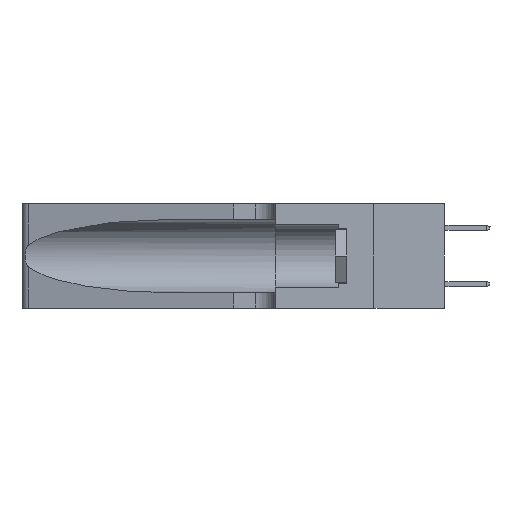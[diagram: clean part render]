
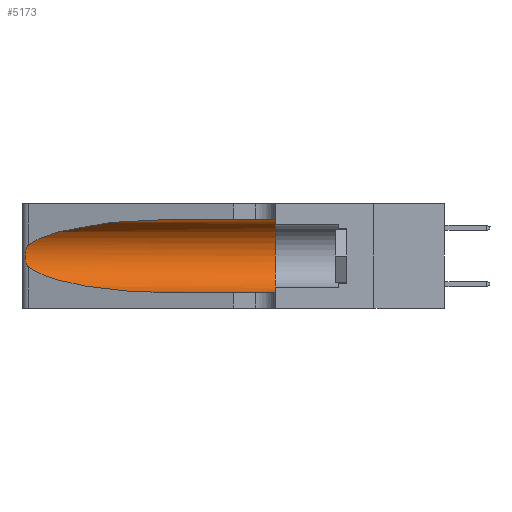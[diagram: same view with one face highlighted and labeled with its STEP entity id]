
A CAD part, left-side view. The second image highlights one B-rep face of the part: STEP entity #5173.
In plain terms, the highlighted cylindrical face has radius 3.308 mm (diameter 6.617 mm), a partial arc.
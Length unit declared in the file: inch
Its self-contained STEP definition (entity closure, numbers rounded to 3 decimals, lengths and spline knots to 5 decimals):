
#245 = VERTEX_POINT ( 'NONE', #17041 ) ;
#412 = CARTESIAN_POINT ( 'NONE',  ( 0.1305, 0.72297, 0.31525 ) ) ;
#603 = CARTESIAN_POINT ( 'NONE',  ( 0.18966, 0.96281, 0.31525 ) ) ;
#1025 = EDGE_CURVE ( 'NONE', #10154, #25639, #23962, .T. ) ;
#1091 = ORIENTED_EDGE ( 'NONE', *, *, #13620, .T. ) ;
#1200 = VERTEX_POINT ( 'NONE', #18886 ) ;
#3694 = ORIENTED_EDGE ( 'NONE', *, *, #9353, .F. ) ;
#4111 = CARTESIAN_POINT ( 'NONE',  ( 0.2373, 1.15595, 0.28018 ) ) ;
#4415 = EDGE_LOOP ( 'NONE', ( #15266, #1091, #21911, #19880, #3694, #12439 ) ) ;
#4439 =( BOUNDED_CURVE ( )  B_SPLINE_CURVE ( 3, ( #412, #603, #4111, #14765 ),
 .UNSPECIFIED., .F., .T. ) 
 B_SPLINE_CURVE_WITH_KNOTS ( ( 4, 4 ),
 ( 1.5708, 2.84003 ),
 .UNSPECIFIED. ) 
 CURVE ( )  GEOMETRIC_REPRESENTATION_ITEM ( )  RATIONAL_B_SPLINE_CURVE ( ( 1., 0.87, 0.87, 1. ) ) 
 REPRESENTATION_ITEM ( '' )  );
#4692 = CARTESIAN_POINT ( 'NONE',  ( 0.25487, 1.22718, 0.14631 ) ) ;
#4801 = DIRECTION ( 'NONE',  ( 0., -1., 0. ) ) ;
#4947 = DIRECTION ( 'NONE',  ( 0., 1., 0. ) ) ;
#5173 = ADVANCED_FACE ( 'NONE', ( #12043 ), #23698, .F. ) ;
#6164 = CARTESIAN_POINT ( 'NONE',  ( 0.25555, 1.22994, 0.2215 ) ) ;
#6769 = CARTESIAN_POINT ( 'NONE',  ( 0.25789, 1.23486, 0.15765 ) ) ;
#6972 = AXIS2_PLACEMENT_3D ( 'NONE', #19323, #9574, #13433 ) ;
#6997 = DIRECTION ( 'NONE',  ( 0., 0., 1. ) ) ;
#7143 = CARTESIAN_POINT ( 'NONE',  ( 0.25487, 1.22718, 0.14631 ) ) ;
#8436 = CARTESIAN_POINT ( 'NONE',  ( 0.1305, 0.72297, 0.05475 ) ) ;
#8871 = VECTOR ( 'NONE', #10184, 39.37008 ) ;
#9102 = EDGE_CURVE ( 'NONE', #1200, #13013, #21924, .T. ) ;
#9353 = EDGE_CURVE ( 'NONE', #25639, #245, #18179, .T. ) ;
#9574 = DIRECTION ( 'NONE',  ( 0., -1., 0. ) ) ;
#10154 = VERTEX_POINT ( 'NONE', #18970 ) ;
#10184 = DIRECTION ( 'NONE',  ( 0., -1., 0. ) ) ;
#10391 = CARTESIAN_POINT ( 'NONE',  ( 0.26075, 1.23896, 0.178 ) ) ;
#11230 = CARTESIAN_POINT ( 'NONE',  ( 0.1305, 0.35, 0.185 ) ) ;
#12031 = LINE ( 'NONE', #14845, #21479 ) ;
#12043 = FACE_OUTER_BOUND ( 'NONE', #4415, .T. ) ;
#12439 = ORIENTED_EDGE ( 'NONE', *, *, #1025, .F. ) ;
#12564 = B_SPLINE_CURVE_WITH_KNOTS ( 'NONE', 3,
 ( #22095, #6164, #17876, #21928, #14335, #16409, #24387, #10391, #18471, #20492, #6769, #17044, #22994, #7143 ),
 .UNSPECIFIED., .F., .F.,
 ( 4, 2, 2, 2, 2, 2, 4 ),
 ( 0., 0.00027, 0.00053, 0.00107, 0.0016, 0.00187, 0.00214 ),
 .UNSPECIFIED. ) ;
#13013 = VERTEX_POINT ( 'NONE', #8436 ) ;
#13024 = CARTESIAN_POINT ( 'NONE',  ( 0.2373, 1.15595, 0.08982 ) ) ;
#13352 = EDGE_CURVE ( 'NONE', #13013, #245, #12031, .T. ) ;
#13433 = DIRECTION ( 'NONE',  ( 0., 0., -1. ) ) ;
#13620 = EDGE_CURVE ( 'NONE', #22296, #1200, #12564, .T. ) ;
#14335 = CARTESIAN_POINT ( 'NONE',  ( 0.25854, 1.2359, 0.20912 ) ) ;
#14416 = CARTESIAN_POINT ( 'NONE',  ( 0.1305, 0.35, 0.31525 ) ) ;
#14433 = AXIS2_PLACEMENT_3D ( 'NONE', #11230, #4947, #6997 ) ;
#14690 = EDGE_CURVE ( 'NONE', #10154, #22296, #4439, .T. ) ;
#14765 = CARTESIAN_POINT ( 'NONE',  ( 0.25487, 1.22718, 0.22369 ) ) ;
#14816 = CARTESIAN_POINT ( 'NONE',  ( 0.25487, 1.22718, 0.22369 ) ) ;
#14845 = CARTESIAN_POINT ( 'NONE',  ( 0.1305, 1.61858, 0.05475 ) ) ;
#15266 = ORIENTED_EDGE ( 'NONE', *, *, #14690, .T. ) ;
#16409 = CARTESIAN_POINT ( 'NONE',  ( 0.26018, 1.23835, 0.19895 ) ) ;
#17041 = CARTESIAN_POINT ( 'NONE',  ( 0.1305, 0.35, 0.05475 ) ) ;
#17044 = CARTESIAN_POINT ( 'NONE',  ( 0.25639, 1.23186, 0.15144 ) ) ;
#17876 = CARTESIAN_POINT ( 'NONE',  ( 0.25639, 1.23184, 0.21858 ) ) ;
#18179 = CIRCLE ( 'NONE', #14433, 0.13025 ) ;
#18471 = CARTESIAN_POINT ( 'NONE',  ( 0.26017, 1.23833, 0.17102 ) ) ;
#18886 = CARTESIAN_POINT ( 'NONE',  ( 0.25487, 1.22718, 0.14631 ) ) ;
#18970 = CARTESIAN_POINT ( 'NONE',  ( 0.1305, 0.72297, 0.31525 ) ) ;
#19323 = CARTESIAN_POINT ( 'NONE',  ( 0.1305, 1.61858, 0.185 ) ) ;
#19880 = ORIENTED_EDGE ( 'NONE', *, *, #13352, .T. ) ;
#19953 = CARTESIAN_POINT ( 'NONE',  ( 0.18966, 0.96281, 0.05475 ) ) ;
#20197 = CARTESIAN_POINT ( 'NONE',  ( 0.1305, 1.61858, 0.31525 ) ) ;
#20492 = CARTESIAN_POINT ( 'NONE',  ( 0.25856, 1.23593, 0.16098 ) ) ;
#21479 = VECTOR ( 'NONE', #4801, 39.37008 ) ;
#21911 = ORIENTED_EDGE ( 'NONE', *, *, #9102, .T. ) ;
#21924 =( BOUNDED_CURVE ( )  B_SPLINE_CURVE ( 3, ( #4692, #13024, #19953, #26070 ),
 .UNSPECIFIED., .F., .T. ) 
 B_SPLINE_CURVE_WITH_KNOTS ( ( 4, 4 ),
 ( 3.44316, 4.71239 ),
 .UNSPECIFIED. ) 
 CURVE ( )  GEOMETRIC_REPRESENTATION_ITEM ( )  RATIONAL_B_SPLINE_CURVE ( ( 1., 0.87, 0.87, 1. ) ) 
 REPRESENTATION_ITEM ( '' )  );
#21928 = CARTESIAN_POINT ( 'NONE',  ( 0.25787, 1.23484, 0.2124 ) ) ;
#22095 = CARTESIAN_POINT ( 'NONE',  ( 0.25487, 1.22718, 0.22369 ) ) ;
#22296 = VERTEX_POINT ( 'NONE', #14816 ) ;
#22994 = CARTESIAN_POINT ( 'NONE',  ( 0.25555, 1.22993, 0.14849 ) ) ;
#23698 = CYLINDRICAL_SURFACE ( 'NONE', #6972, 0.13025 ) ;
#23962 = LINE ( 'NONE', #20197, #8871 ) ;
#24387 = CARTESIAN_POINT ( 'NONE',  ( 0.26075, 1.23896, 0.19203 ) ) ;
#25639 = VERTEX_POINT ( 'NONE', #14416 ) ;
#26070 = CARTESIAN_POINT ( 'NONE',  ( 0.1305, 0.72297, 0.05475 ) ) ;
